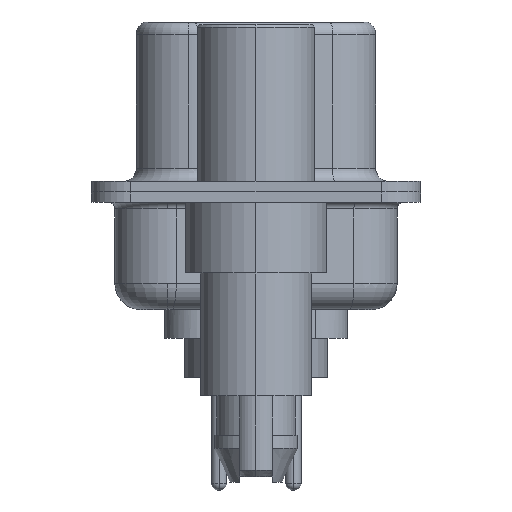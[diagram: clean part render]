
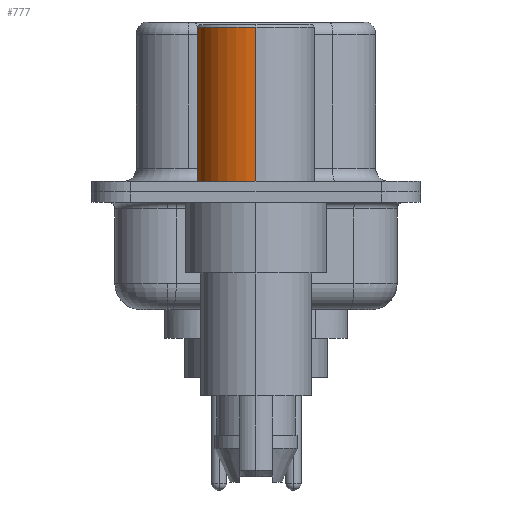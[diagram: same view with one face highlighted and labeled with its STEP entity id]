
A CAD part, left-side view. The second image highlights one B-rep face of the part: STEP entity #777.
In plain terms, the highlighted cylindrical face has radius 2.25 mm (diameter 4.5 mm), a partial arc.
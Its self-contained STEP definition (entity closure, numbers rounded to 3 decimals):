
#214 = CYLINDRICAL_SURFACE ( 'NONE', #10267, 2.25 ) ;
#682 = DIRECTION ( 'NONE',  ( 0., 0., 1. ) ) ;
#777 = ADVANCED_FACE ( 'NONE', ( #15205 ), #214, .T. ) ;
#1621 = AXIS2_PLACEMENT_3D ( 'NONE', #9986, #9594, #9577 ) ;
#1644 = AXIS2_PLACEMENT_3D ( 'NONE', #15823, #682, #10730 ) ;
#1677 = CARTESIAN_POINT ( 'NONE',  ( 0., 0., 0.581 ) ) ;
#2113 = CARTESIAN_POINT ( 'NONE',  ( 2.25, 0., 0.581 ) ) ;
#2558 = ORIENTED_EDGE ( 'NONE', *, *, #6786, .F. ) ;
#3012 = CARTESIAN_POINT ( 'NONE',  ( 2.25, 0., 0.4 ) ) ;
#3270 = DIRECTION ( 'NONE',  ( 1., 0., 0. ) ) ;
#3391 = CARTESIAN_POINT ( 'NONE',  ( -2.25, 0., 0.4 ) ) ;
#6143 = VECTOR ( 'NONE', #9051, 1000. ) ;
#6534 = DIRECTION ( 'NONE',  ( 0., 0., 1. ) ) ;
#6575 = CIRCLE ( 'NONE', #1621, 2.25 ) ;
#6614 = EDGE_CURVE ( 'NONE', #6824, #16486, #7921, .T. ) ;
#6702 = EDGE_CURVE ( 'NONE', #10879, #15731, #6575, .T. ) ;
#6703 = EDGE_CURVE ( 'NONE', #15731, #16486, #10349, .T. ) ;
#6708 = ORIENTED_EDGE ( 'NONE', *, *, #6703, .T. ) ;
#6786 = EDGE_CURVE ( 'NONE', #10879, #6824, #13651, .T. ) ;
#6824 = VERTEX_POINT ( 'NONE', #10498 ) ;
#7486 = ORIENTED_EDGE ( 'NONE', *, *, #6702, .T. ) ;
#7921 = CIRCLE ( 'NONE', #1644, 2.25 ) ;
#8877 = ORIENTED_EDGE ( 'NONE', *, *, #6614, .F. ) ;
#9046 = DIRECTION ( 'NONE',  ( 0., 0., 1. ) ) ;
#9051 = DIRECTION ( 'NONE',  ( 0., 0., 1. ) ) ;
#9577 = DIRECTION ( 'NONE',  ( 1., 0., 0. ) ) ;
#9594 = DIRECTION ( 'NONE',  ( 0., 0., 1. ) ) ;
#9986 = CARTESIAN_POINT ( 'NONE',  ( 0., 0., 0.4 ) ) ;
#10267 = AXIS2_PLACEMENT_3D ( 'NONE', #1677, #9046, #3270 ) ;
#10268 = CARTESIAN_POINT ( 'NONE',  ( -2.25, 0., 0.581 ) ) ;
#10349 = LINE ( 'NONE', #10268, #6143 ) ;
#10498 = CARTESIAN_POINT ( 'NONE',  ( 2.25, 0., 6.3 ) ) ;
#10730 = DIRECTION ( 'NONE',  ( 1., 0., 0. ) ) ;
#10879 = VERTEX_POINT ( 'NONE', #3012 ) ;
#13651 = LINE ( 'NONE', #2113, #16381 ) ;
#15060 = CARTESIAN_POINT ( 'NONE',  ( -2.25, 0., 6.3 ) ) ;
#15205 = FACE_OUTER_BOUND ( 'NONE', #15249, .T. ) ;
#15249 = EDGE_LOOP ( 'NONE', ( #7486, #6708, #8877, #2558 ) ) ;
#15731 = VERTEX_POINT ( 'NONE', #3391 ) ;
#15823 = CARTESIAN_POINT ( 'NONE',  ( 0., 0., 6.3 ) ) ;
#16381 = VECTOR ( 'NONE', #6534, 1000. ) ;
#16486 = VERTEX_POINT ( 'NONE', #15060 ) ;
